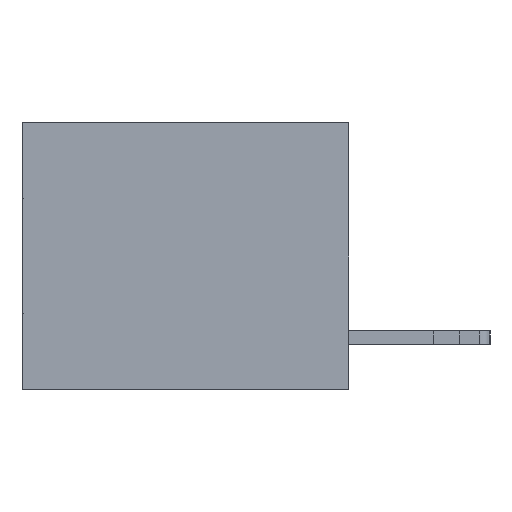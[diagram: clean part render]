
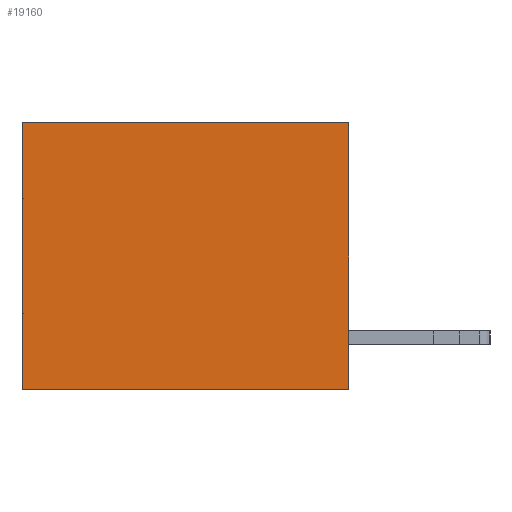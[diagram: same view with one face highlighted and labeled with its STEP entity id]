
A CAD part, left-side view. The second image highlights one B-rep face of the part: STEP entity #19160.
In plain terms, the highlighted planar face has unit normal (-1, 0, 0).
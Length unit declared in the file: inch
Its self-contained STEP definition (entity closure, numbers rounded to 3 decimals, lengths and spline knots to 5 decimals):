
#310 = ORIENTED_EDGE ( 'NONE', *, *, #14143, .T. ) ;
#401 = LINE ( 'NONE', #8269, #8125 ) ;
#431 = EDGE_CURVE ( 'NONE', #6466, #22199, #8770, .T. ) ;
#472 = CARTESIAN_POINT ( 'NONE',  ( 0.3165, 0., -0.49 ) ) ;
#544 = ORIENTED_EDGE ( 'NONE', *, *, #3699, .F. ) ;
#650 = VECTOR ( 'NONE', #28366, 39.37008 ) ;
#1267 = ORIENTED_EDGE ( 'NONE', *, *, #431, .F. ) ;
#2314 = EDGE_LOOP ( 'NONE', ( #17254, #1267, #544, #310 ) ) ;
#2470 = CARTESIAN_POINT ( 'NONE',  ( 0.3165, 0.6, 0. ) ) ;
#2840 = EDGE_CURVE ( 'NONE', #13067, #22199, #31854, .T. ) ;
#3389 = CARTESIAN_POINT ( 'NONE',  ( 0.3165, 0., -0.49 ) ) ;
#3699 = EDGE_CURVE ( 'NONE', #29770, #6466, #401, .T. ) ;
#4731 = DIRECTION ( 'NONE',  ( 0., 0., -1. ) ) ;
#6466 = VERTEX_POINT ( 'NONE', #472 ) ;
#8125 = VECTOR ( 'NONE', #18163, 39.37008 ) ;
#8269 = CARTESIAN_POINT ( 'NONE',  ( 0.3165, 0., -0.49 ) ) ;
#8770 = LINE ( 'NONE', #3389, #650 ) ;
#10461 = CARTESIAN_POINT ( 'NONE',  ( 0.3165, 0.6, -0.49 ) ) ;
#10826 = DIRECTION ( 'NONE',  ( 1., 0., 0. ) ) ;
#11031 = CARTESIAN_POINT ( 'NONE',  ( 0.3165, 0., -0.49 ) ) ;
#13067 = VERTEX_POINT ( 'NONE', #2470 ) ;
#14143 = EDGE_CURVE ( 'NONE', #29770, #13067, #27387, .T. ) ;
#14278 = VECTOR ( 'NONE', #18492, 39.37008 ) ;
#15636 = PLANE ( 'NONE',  #19086 ) ;
#15914 = CARTESIAN_POINT ( 'NONE',  ( 0.3165, 0., 0. ) ) ;
#17254 = ORIENTED_EDGE ( 'NONE', *, *, #2840, .T. ) ;
#17889 = CARTESIAN_POINT ( 'NONE',  ( 0.3165, 0., 0. ) ) ;
#18163 = DIRECTION ( 'NONE',  ( 0., 0., -1. ) ) ;
#18492 = DIRECTION ( 'NONE',  ( 0., 1., 0. ) ) ;
#19086 = AXIS2_PLACEMENT_3D ( 'NONE', #11031, #10826, #30660 ) ;
#19160 = ADVANCED_FACE ( 'NONE', ( #22086 ), #15636, .F. ) ;
#22086 = FACE_OUTER_BOUND ( 'NONE', #2314, .T. ) ;
#22199 = VERTEX_POINT ( 'NONE', #10461 ) ;
#27387 = LINE ( 'NONE', #15914, #14278 ) ;
#28366 = DIRECTION ( 'NONE',  ( 0., 1., 0. ) ) ;
#29548 = VECTOR ( 'NONE', #4731, 39.37008 ) ;
#29770 = VERTEX_POINT ( 'NONE', #17889 ) ;
#30660 = DIRECTION ( 'NONE',  ( 0., 0., -1. ) ) ;
#31617 = CARTESIAN_POINT ( 'NONE',  ( 0.3165, 0.6, -0.49 ) ) ;
#31854 = LINE ( 'NONE', #31617, #29548 ) ;
